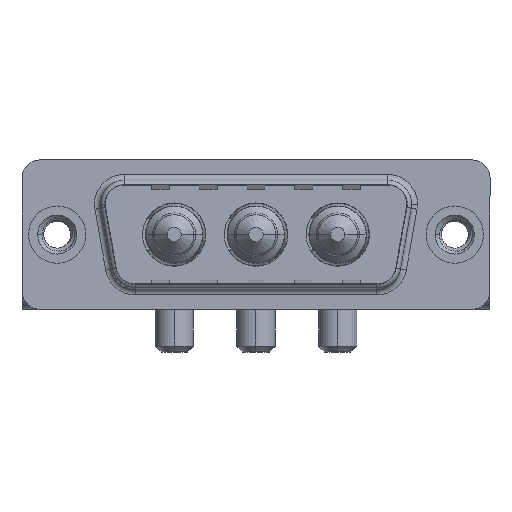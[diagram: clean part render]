
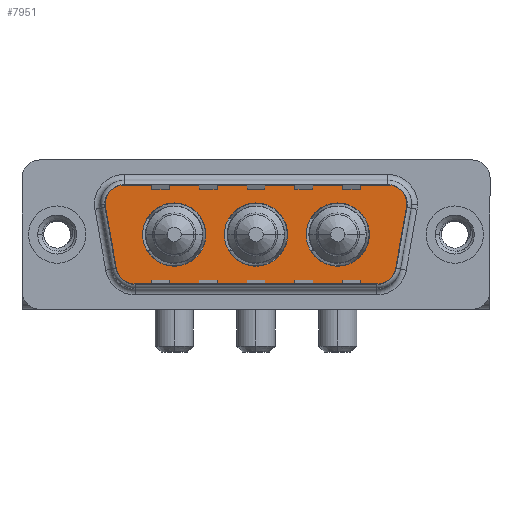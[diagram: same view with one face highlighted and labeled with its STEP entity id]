
A CAD part, top view. The second image highlights one B-rep face of the part: STEP entity #7951.
In plain terms, the highlighted planar face has unit normal (0, 0, 1).
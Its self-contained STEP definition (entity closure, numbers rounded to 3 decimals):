
#102 = VERTEX_POINT ( 'NONE', #5179 ) ;
#404 = ORIENTED_EDGE ( 'NONE', *, *, #4095, .F. ) ;
#699 = VERTEX_POINT ( 'NONE', #6530 ) ;
#728 = EDGE_CURVE ( 'NONE', #11327, #102, #3430, .T. ) ;
#739 = ORIENTED_EDGE ( 'NONE', *, *, #13344, .T. ) ;
#922 = VERTEX_POINT ( 'NONE', #4611 ) ;
#1076 = LINE ( 'NONE', #5291, #1705 ) ;
#1184 = EDGE_CURVE ( 'NONE', #4397, #13453, #9368, .T. ) ;
#1310 = DIRECTION ( 'NONE',  ( 0., 0., 1. ) ) ;
#1367 = EDGE_LOOP ( 'NONE', ( #10106, #6880 ) ) ;
#1705 = VECTOR ( 'NONE', #9508, 1000. ) ;
#1750 = DIRECTION ( 'NONE',  ( 0., 0., 1. ) ) ;
#1802 = ORIENTED_EDGE ( 'NONE', *, *, #10913, .T. ) ;
#1840 = FACE_BOUND ( 'NONE', #1367, .T. ) ;
#2000 = CARTESIAN_POINT ( 'NONE',  ( 23.5, 0., 0. ) ) ;
#2004 = VERTEX_POINT ( 'NONE', #6468 ) ;
#2061 = ORIENTED_EDGE ( 'NONE', *, *, #4873, .F. ) ;
#2201 = CARTESIAN_POINT ( 'NONE',  ( 20.85, 0., 0. ) ) ;
#2411 = CIRCLE ( 'NONE', #8624, 2.65 ) ;
#2459 = DIRECTION ( 'NONE',  ( 1., 0., 0. ) ) ;
#2687 = DIRECTION ( 'NONE',  ( 0., 0., 1. ) ) ;
#2778 = DIRECTION ( 'NONE',  ( 1., 0., 0. ) ) ;
#2805 = CARTESIAN_POINT ( 'NONE',  ( 26.866, -2.9, 0. ) ) ;
#2832 = CIRCLE ( 'NONE', #11205, 2. ) ;
#2845 = AXIS2_PLACEMENT_3D ( 'NONE', #13521, #10358, #6206 ) ;
#2875 = EDGE_CURVE ( 'NONE', #11690, #5761, #2411, .T. ) ;
#3018 = CARTESIAN_POINT ( 'NONE',  ( 7.15, 0., 0. ) ) ;
#3078 = FACE_BOUND ( 'NONE', #13421, .T. ) ;
#3337 = DIRECTION ( 'NONE',  ( 0., 0., 1. ) ) ;
#3343 = CARTESIAN_POINT ( 'NONE',  ( 3.441, 2.553, 0. ) ) ;
#3421 = ORIENTED_EDGE ( 'NONE', *, *, #11525, .T. ) ;
#3430 = LINE ( 'NONE', #8759, #10240 ) ;
#3528 = VERTEX_POINT ( 'NONE', #9545 ) ;
#3640 = CARTESIAN_POINT ( 'NONE',  ( 5.411, 2.9, 0. ) ) ;
#3683 = AXIS2_PLACEMENT_3D ( 'NONE', #7999, #8141, #9938 ) ;
#3879 = ORIENTED_EDGE ( 'NONE', *, *, #10706, .T. ) ;
#4001 = VERTEX_POINT ( 'NONE', #13527 ) ;
#4095 = EDGE_CURVE ( 'NONE', #2004, #3528, #5895, .T. ) ;
#4329 = CARTESIAN_POINT ( 'NONE',  ( 6.434, -4.9, 0. ) ) ;
#4397 = VERTEX_POINT ( 'NONE', #3018 ) ;
#4566 = ORIENTED_EDGE ( 'NONE', *, *, #9813, .T. ) ;
#4611 = CARTESIAN_POINT ( 'NONE',  ( 6.434, -4.9, 0. ) ) ;
#4782 = CIRCLE ( 'NONE', #3683, 2. ) ;
#4839 = DIRECTION ( 'NONE',  ( 0., 0., 1. ) ) ;
#4873 = EDGE_CURVE ( 'NONE', #13453, #4397, #5886, .T. ) ;
#5070 = CIRCLE ( 'NONE', #12762, 2. ) ;
#5179 = CARTESIAN_POINT ( 'NONE',  ( 5.411, 4.9, 0. ) ) ;
#5187 = ORIENTED_EDGE ( 'NONE', *, *, #7859, .T. ) ;
#5261 = AXIS2_PLACEMENT_3D ( 'NONE', #7116, #4839, #13183 ) ;
#5265 = VERTEX_POINT ( 'NONE', #11190 ) ;
#5291 = CARTESIAN_POINT ( 'NONE',  ( 29.859, 2.553, 0. ) ) ;
#5628 = ORIENTED_EDGE ( 'NONE', *, *, #728, .T. ) ;
#5761 = VERTEX_POINT ( 'NONE', #5995 ) ;
#5886 = CIRCLE ( 'NONE', #13374, 2.65 ) ;
#5895 = CIRCLE ( 'NONE', #7876, 2.65 ) ;
#5995 = CARTESIAN_POINT ( 'NONE',  ( 26.15, 0., 0. ) ) ;
#6063 = CARTESIAN_POINT ( 'NONE',  ( 12.45, 0., 0. ) ) ;
#6144 = DIRECTION ( 'NONE',  ( 0., 0., 1. ) ) ;
#6206 = DIRECTION ( 'NONE',  ( -1., 0., 0. ) ) ;
#6468 = CARTESIAN_POINT ( 'NONE',  ( 19.3, 0., 0. ) ) ;
#6494 = CARTESIAN_POINT ( 'NONE',  ( 9.8, 0., 0. ) ) ;
#6500 = LINE ( 'NONE', #3343, #11627 ) ;
#6530 = CARTESIAN_POINT ( 'NONE',  ( 26.866, -4.9, 0. ) ) ;
#6532 = VECTOR ( 'NONE', #9658, 1000. ) ;
#6573 = VERTEX_POINT ( 'NONE', #6796 ) ;
#6796 = CARTESIAN_POINT ( 'NONE',  ( 29.889, 2.9, 0. ) ) ;
#6880 = ORIENTED_EDGE ( 'NONE', *, *, #2875, .F. ) ;
#6949 = DIRECTION ( 'NONE',  ( 0., 0., 1. ) ) ;
#7009 = ORIENTED_EDGE ( 'NONE', *, *, #1184, .F. ) ;
#7116 = CARTESIAN_POINT ( 'NONE',  ( 6.434, -2.9, 0. ) ) ;
#7157 = DIRECTION ( 'NONE',  ( 0., 0., 1. ) ) ;
#7433 = EDGE_CURVE ( 'NONE', #3528, #2004, #9690, .T. ) ;
#7472 = CIRCLE ( 'NONE', #13645, 2.65 ) ;
#7558 = DIRECTION ( 'NONE',  ( 0., 0., 1. ) ) ;
#7859 = EDGE_CURVE ( 'NONE', #102, #9280, #5070, .T. ) ;
#7876 = AXIS2_PLACEMENT_3D ( 'NONE', #11859, #1310, #10838 ) ;
#7951 = ADVANCED_FACE ( 'NONE', ( #12256, #1840, #3078, #8204 ), #8263, .T. ) ;
#7999 = CARTESIAN_POINT ( 'NONE',  ( 27.889, 2.9, 0. ) ) ;
#8131 = CARTESIAN_POINT ( 'NONE',  ( 23.5, 0., 0. ) ) ;
#8141 = DIRECTION ( 'NONE',  ( 0., 0., 1. ) ) ;
#8191 = EDGE_LOOP ( 'NONE', ( #1802, #4566, #3421, #11189, #5628, #5187, #3879, #739, #12265 ) ) ;
#8204 = FACE_OUTER_BOUND ( 'NONE', #8191, .T. ) ;
#8263 = PLANE ( 'NONE',  #9480 ) ;
#8383 = ORIENTED_EDGE ( 'NONE', *, *, #7433, .F. ) ;
#8497 = CARTESIAN_POINT ( 'NONE',  ( 27.889, 4.9, 0. ) ) ;
#8624 = AXIS2_PLACEMENT_3D ( 'NONE', #8131, #7157, #13500 ) ;
#8713 = EDGE_LOOP ( 'NONE', ( #404, #8383 ) ) ;
#8759 = CARTESIAN_POINT ( 'NONE',  ( 5.411, 4.9, 0. ) ) ;
#8806 = CIRCLE ( 'NONE', #2845, 2. ) ;
#9280 = VERTEX_POINT ( 'NONE', #13656 ) ;
#9368 = CIRCLE ( 'NONE', #12884, 2.65 ) ;
#9480 = AXIS2_PLACEMENT_3D ( 'NONE', #2805, #11231, #12462 ) ;
#9508 = DIRECTION ( 'NONE',  ( 0.174, 0.985, 0. ) ) ;
#9513 = EDGE_CURVE ( 'NONE', #922, #699, #11777, .T. ) ;
#9545 = CARTESIAN_POINT ( 'NONE',  ( 14., 0., 0. ) ) ;
#9574 = EDGE_CURVE ( 'NONE', #6573, #11327, #4782, .T. ) ;
#9658 = DIRECTION ( 'NONE',  ( 1., 0., 0. ) ) ;
#9690 = CIRCLE ( 'NONE', #13441, 2.65 ) ;
#9750 = CARTESIAN_POINT ( 'NONE',  ( 29.859, 2.553, 0. ) ) ;
#9813 = EDGE_CURVE ( 'NONE', #5265, #11240, #1076, .T. ) ;
#9873 = DIRECTION ( 'NONE',  ( 1., 0., 0. ) ) ;
#9938 = DIRECTION ( 'NONE',  ( -1., 0., 0. ) ) ;
#10106 = ORIENTED_EDGE ( 'NONE', *, *, #11908, .F. ) ;
#10240 = VECTOR ( 'NONE', #12740, 1000. ) ;
#10358 = DIRECTION ( 'NONE',  ( 0., 0., 1. ) ) ;
#10419 = DIRECTION ( 'NONE',  ( 1., 0., 0. ) ) ;
#10706 = EDGE_CURVE ( 'NONE', #9280, #4001, #6500, .T. ) ;
#10713 = DIRECTION ( 'NONE',  ( 1., 0., 0. ) ) ;
#10719 = DIRECTION ( 'NONE',  ( 0.174, -0.985, 0. ) ) ;
#10838 = DIRECTION ( 'NONE',  ( 1., 0., 0. ) ) ;
#10913 = EDGE_CURVE ( 'NONE', #699, #5265, #2832, .T. ) ;
#11189 = ORIENTED_EDGE ( 'NONE', *, *, #9574, .T. ) ;
#11190 = CARTESIAN_POINT ( 'NONE',  ( 28.836, -3.247, 0. ) ) ;
#11205 = AXIS2_PLACEMENT_3D ( 'NONE', #12168, #1750, #2778 ) ;
#11231 = DIRECTION ( 'NONE',  ( 0., 0., 1. ) ) ;
#11240 = VERTEX_POINT ( 'NONE', #9750 ) ;
#11327 = VERTEX_POINT ( 'NONE', #8497 ) ;
#11525 = EDGE_CURVE ( 'NONE', #11240, #6573, #8806, .T. ) ;
#11627 = VECTOR ( 'NONE', #10719, 1000. ) ;
#11690 = VERTEX_POINT ( 'NONE', #2201 ) ;
#11760 = DIRECTION ( 'NONE',  ( 1., 0., 0. ) ) ;
#11777 = LINE ( 'NONE', #4329, #6532 ) ;
#11859 = CARTESIAN_POINT ( 'NONE',  ( 16.65, 0., 0. ) ) ;
#11876 = CIRCLE ( 'NONE', #5261, 2. ) ;
#11908 = EDGE_CURVE ( 'NONE', #5761, #11690, #7472, .T. ) ;
#12142 = CARTESIAN_POINT ( 'NONE',  ( 16.65, 0., 0. ) ) ;
#12168 = CARTESIAN_POINT ( 'NONE',  ( 26.866, -2.9, 0. ) ) ;
#12256 = FACE_BOUND ( 'NONE', #8713, .T. ) ;
#12265 = ORIENTED_EDGE ( 'NONE', *, *, #9513, .T. ) ;
#12462 = DIRECTION ( 'NONE',  ( 1., 0., 0. ) ) ;
#12650 = CARTESIAN_POINT ( 'NONE',  ( 9.8, 0., 0. ) ) ;
#12740 = DIRECTION ( 'NONE',  ( -1., 0., 0. ) ) ;
#12762 = AXIS2_PLACEMENT_3D ( 'NONE', #3640, #6949, #2459 ) ;
#12884 = AXIS2_PLACEMENT_3D ( 'NONE', #12650, #7558, #11760 ) ;
#13183 = DIRECTION ( 'NONE',  ( -1., 0., 0. ) ) ;
#13344 = EDGE_CURVE ( 'NONE', #4001, #922, #11876, .T. ) ;
#13374 = AXIS2_PLACEMENT_3D ( 'NONE', #6494, #3337, #10713 ) ;
#13421 = EDGE_LOOP ( 'NONE', ( #2061, #7009 ) ) ;
#13441 = AXIS2_PLACEMENT_3D ( 'NONE', #12142, #2687, #9873 ) ;
#13453 = VERTEX_POINT ( 'NONE', #6063 ) ;
#13500 = DIRECTION ( 'NONE',  ( 1., 0., 0. ) ) ;
#13521 = CARTESIAN_POINT ( 'NONE',  ( 27.889, 2.9, 0. ) ) ;
#13527 = CARTESIAN_POINT ( 'NONE',  ( 4.464, -3.247, 0. ) ) ;
#13645 = AXIS2_PLACEMENT_3D ( 'NONE', #2000, #6144, #10419 ) ;
#13656 = CARTESIAN_POINT ( 'NONE',  ( 3.441, 2.553, 0. ) ) ;
